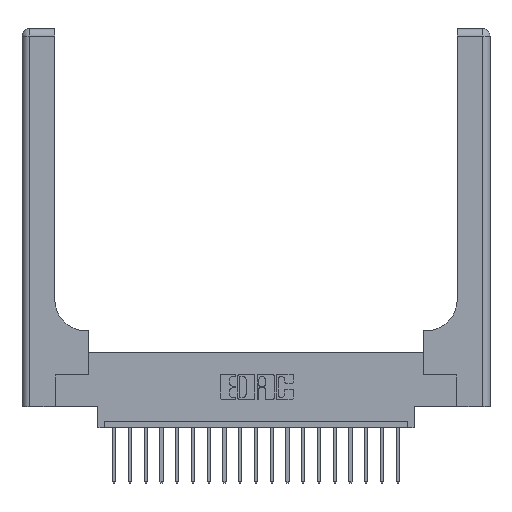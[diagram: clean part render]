
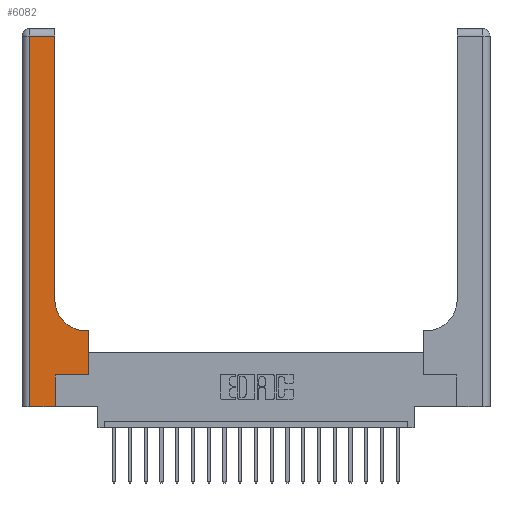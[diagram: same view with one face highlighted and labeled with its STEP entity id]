
A CAD part, top view. The second image highlights one B-rep face of the part: STEP entity #6082.
In plain terms, the highlighted planar face has unit normal (0, 0, 1).
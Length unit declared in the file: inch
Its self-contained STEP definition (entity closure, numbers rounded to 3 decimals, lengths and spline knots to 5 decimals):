
#326 = EDGE_LOOP ( 'NONE', ( #15039, #9484, #5366, #737, #7277, #6286, #5654, #3441, #13214 ) ) ;
#383 = DIRECTION ( 'NONE',  ( 1., 0., 0. ) ) ;
#737 = ORIENTED_EDGE ( 'NONE', *, *, #17093, .T. ) ;
#880 = VERTEX_POINT ( 'NONE', #5647 ) ;
#955 = DIRECTION ( 'NONE',  ( -1., 0., 0. ) ) ;
#1424 = CARTESIAN_POINT ( 'NONE',  ( 0.06, 0., 0.37 ) ) ;
#1535 = VERTEX_POINT ( 'NONE', #16702 ) ;
#2942 = VERTEX_POINT ( 'NONE', #16527 ) ;
#3150 = EDGE_CURVE ( 'NONE', #7069, #8941, #16433, .T. ) ;
#3328 = LINE ( 'NONE', #20085, #4766 ) ;
#3441 = ORIENTED_EDGE ( 'NONE', *, *, #3925, .T. ) ;
#3684 = DIRECTION ( 'NONE',  ( -1., 0., 0. ) ) ;
#3925 = EDGE_CURVE ( 'NONE', #10883, #7069, #18120, .T. ) ;
#4038 = LINE ( 'NONE', #12099, #8639 ) ;
#4359 = DIRECTION ( 'NONE',  ( 1., 0., 0. ) ) ;
#4479 = EDGE_CURVE ( 'NONE', #2942, #13662, #7614, .T. ) ;
#4766 = VECTOR ( 'NONE', #18734, 39.37008 ) ;
#4785 = AXIS2_PLACEMENT_3D ( 'NONE', #16034, #15836, #383 ) ;
#5002 = VECTOR ( 'NONE', #8825, 39.37008 ) ;
#5095 = CARTESIAN_POINT ( 'NONE',  ( 0., 3., 0.37 ) ) ;
#5366 = ORIENTED_EDGE ( 'NONE', *, *, #13880, .T. ) ;
#5647 = CARTESIAN_POINT ( 'NONE',  ( 0.06, 2.94, 0.37 ) ) ;
#5654 = ORIENTED_EDGE ( 'NONE', *, *, #9331, .T. ) ;
#5655 = VECTOR ( 'NONE', #11126, 39.37008 ) ;
#5988 = CARTESIAN_POINT ( 'NONE',  ( 0.26, 0.85, 0.37 ) ) ;
#6082 = ADVANCED_FACE ( 'NONE', ( #19502 ), #11542, .F. ) ;
#6105 = VERTEX_POINT ( 'NONE', #16266 ) ;
#6286 = ORIENTED_EDGE ( 'NONE', *, *, #4479, .T. ) ;
#6722 = CARTESIAN_POINT ( 'NONE',  ( 0.265, 0., 0.37 ) ) ;
#7069 = VERTEX_POINT ( 'NONE', #8822 ) ;
#7277 = ORIENTED_EDGE ( 'NONE', *, *, #9479, .T. ) ;
#7614 = LINE ( 'NONE', #12367, #17869 ) ;
#8109 = CARTESIAN_POINT ( 'NONE',  ( 0.528, 0.25, 0.37 ) ) ;
#8639 = VECTOR ( 'NONE', #4359, 39.37008 ) ;
#8822 = CARTESIAN_POINT ( 'NONE',  ( 0.51, 0.6, 0.37 ) ) ;
#8825 = DIRECTION ( 'NONE',  ( -1., 0., 0. ) ) ;
#8907 = EDGE_CURVE ( 'NONE', #8941, #1535, #3328, .T. ) ;
#8941 = VERTEX_POINT ( 'NONE', #5988 ) ;
#9331 = EDGE_CURVE ( 'NONE', #13662, #10883, #14665, .T. ) ;
#9479 = EDGE_CURVE ( 'NONE', #6105, #2942, #15651, .T. ) ;
#9484 = ORIENTED_EDGE ( 'NONE', *, *, #17070, .T. ) ;
#9872 = VERTEX_POINT ( 'NONE', #1424 ) ;
#10152 = AXIS2_PLACEMENT_3D ( 'NONE', #5095, #15995, #3684 ) ;
#10883 = VERTEX_POINT ( 'NONE', #19755 ) ;
#11126 = DIRECTION ( 'NONE',  ( 0., 1., 0. ) ) ;
#11542 = PLANE ( 'NONE',  #10152 ) ;
#12099 = CARTESIAN_POINT ( 'NONE',  ( 0., 0., 0.37 ) ) ;
#12367 = CARTESIAN_POINT ( 'NONE',  ( 0.265, 0.25, 0.37 ) ) ;
#12726 = CARTESIAN_POINT ( 'NONE',  ( 0.528, 0.25, 0.37 ) ) ;
#12967 = VECTOR ( 'NONE', #17499, 39.37008 ) ;
#13214 = ORIENTED_EDGE ( 'NONE', *, *, #3150, .T. ) ;
#13504 = CARTESIAN_POINT ( 'NONE',  ( 0.06, 3., 0.37 ) ) ;
#13662 = VERTEX_POINT ( 'NONE', #8109 ) ;
#13880 = EDGE_CURVE ( 'NONE', #880, #9872, #19858, .T. ) ;
#14665 = LINE ( 'NONE', #12726, #5655 ) ;
#15039 = ORIENTED_EDGE ( 'NONE', *, *, #8907, .T. ) ;
#15651 = LINE ( 'NONE', #6722, #12967 ) ;
#15728 = VECTOR ( 'NONE', #18203, 39.37008 ) ;
#15836 = DIRECTION ( 'NONE',  ( 0., 0., -1. ) ) ;
#15995 = DIRECTION ( 'NONE',  ( 0., 0., -1. ) ) ;
#16034 = CARTESIAN_POINT ( 'NONE',  ( 0.51, 0.85, 0.37 ) ) ;
#16266 = CARTESIAN_POINT ( 'NONE',  ( 0.265, 0., 0.37 ) ) ;
#16433 = CIRCLE ( 'NONE', #4785, 0.25 ) ;
#16527 = CARTESIAN_POINT ( 'NONE',  ( 0.265, 0.25, 0.37 ) ) ;
#16702 = CARTESIAN_POINT ( 'NONE',  ( 0.26, 2.94, 0.37 ) ) ;
#16824 = CARTESIAN_POINT ( 'NONE',  ( 0., 2.94, 0.37 ) ) ;
#17008 = DIRECTION ( 'NONE',  ( 1., 0., 0. ) ) ;
#17070 = EDGE_CURVE ( 'NONE', #1535, #880, #18901, .T. ) ;
#17093 = EDGE_CURVE ( 'NONE', #9872, #6105, #4038, .T. ) ;
#17390 = VECTOR ( 'NONE', #955, 39.37008 ) ;
#17499 = DIRECTION ( 'NONE',  ( 0., 1., 0. ) ) ;
#17869 = VECTOR ( 'NONE', #17008, 39.37008 ) ;
#18024 = CARTESIAN_POINT ( 'NONE',  ( 0.26, 0.6, 0.37 ) ) ;
#18120 = LINE ( 'NONE', #18024, #17390 ) ;
#18203 = DIRECTION ( 'NONE',  ( 0., -1., 0. ) ) ;
#18734 = DIRECTION ( 'NONE',  ( 0., 1., 0. ) ) ;
#18901 = LINE ( 'NONE', #16824, #5002 ) ;
#19502 = FACE_OUTER_BOUND ( 'NONE', #326, .T. ) ;
#19755 = CARTESIAN_POINT ( 'NONE',  ( 0.528, 0.6, 0.37 ) ) ;
#19858 = LINE ( 'NONE', #13504, #15728 ) ;
#20085 = CARTESIAN_POINT ( 'NONE',  ( 0.26, 3., 0.37 ) ) ;
